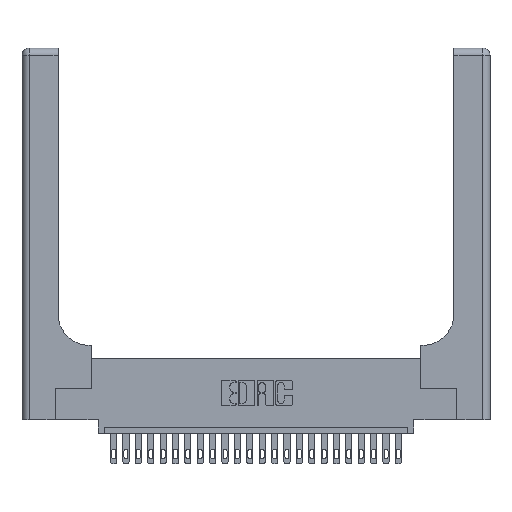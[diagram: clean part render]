
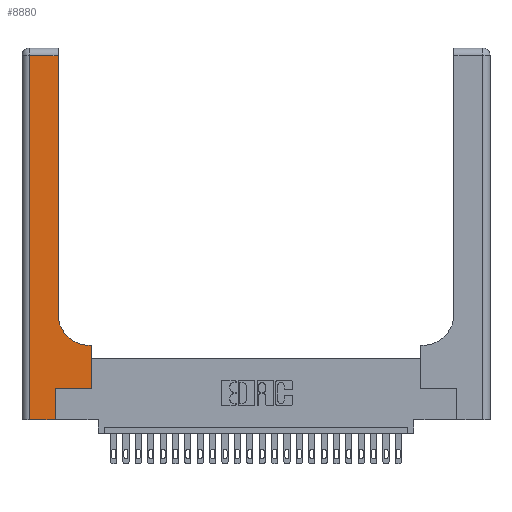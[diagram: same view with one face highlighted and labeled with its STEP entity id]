
A CAD part, top view. The second image highlights one B-rep face of the part: STEP entity #8880.
In plain terms, the highlighted planar face has unit normal (0, 0, 1).
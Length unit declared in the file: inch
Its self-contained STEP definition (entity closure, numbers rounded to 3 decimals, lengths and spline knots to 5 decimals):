
#120 = DIRECTION ( 'NONE',  ( 0., 1., 0. ) ) ;
#512 = ORIENTED_EDGE ( 'NONE', *, *, #14197, .T. ) ;
#911 = VERTEX_POINT ( 'NONE', #7799 ) ;
#1427 = LINE ( 'NONE', #4566, #17618 ) ;
#1475 = LINE ( 'NONE', #22172, #3324 ) ;
#1611 = PLANE ( 'NONE',  #11860 ) ;
#1965 = LINE ( 'NONE', #23813, #8492 ) ;
#2559 = LINE ( 'NONE', #25219, #19685 ) ;
#2937 = CARTESIAN_POINT ( 'NONE',  ( 0.269, 0., 0.37 ) ) ;
#3324 = VECTOR ( 'NONE', #23916, 39.37008 ) ;
#3340 = DIRECTION ( 'NONE',  ( 0., 1., 0. ) ) ;
#3597 = CARTESIAN_POINT ( 'NONE',  ( 0.06, 2.94, 0.37 ) ) ;
#3850 = VERTEX_POINT ( 'NONE', #7795 ) ;
#4311 = DIRECTION ( 'NONE',  ( -1., 0., 0. ) ) ;
#4566 = CARTESIAN_POINT ( 'NONE',  ( 0.5585, 0.25, 0.37 ) ) ;
#5113 = ORIENTED_EDGE ( 'NONE', *, *, #22026, .T. ) ;
#5158 = LINE ( 'NONE', #13811, #24402 ) ;
#5222 = VECTOR ( 'NONE', #4311, 39.37008 ) ;
#5595 = CARTESIAN_POINT ( 'NONE',  ( 0., 3., 0.37 ) ) ;
#5942 = VERTEX_POINT ( 'NONE', #2937 ) ;
#6068 = ORIENTED_EDGE ( 'NONE', *, *, #8853, .T. ) ;
#6918 = CARTESIAN_POINT ( 'NONE',  ( 0.2915, 2.94, 0.37 ) ) ;
#7169 = DIRECTION ( 'NONE',  ( 1., 0., 0. ) ) ;
#7316 = DIRECTION ( 'NONE',  ( 1., 0., 0. ) ) ;
#7342 = VERTEX_POINT ( 'NONE', #24011 ) ;
#7644 = ORIENTED_EDGE ( 'NONE', *, *, #8374, .T. ) ;
#7795 = CARTESIAN_POINT ( 'NONE',  ( 0.5585, 0.25, 0.37 ) ) ;
#7799 = CARTESIAN_POINT ( 'NONE',  ( 0.06, 0., 0.37 ) ) ;
#8374 = EDGE_CURVE ( 'NONE', #11937, #13848, #12466, .T. ) ;
#8492 = VECTOR ( 'NONE', #14011, 39.37008 ) ;
#8853 = EDGE_CURVE ( 'NONE', #5942, #13074, #2559, .T. ) ;
#8880 = ADVANCED_FACE ( 'NONE', ( #17200 ), #1611, .F. ) ;
#8894 = ORIENTED_EDGE ( 'NONE', *, *, #12734, .T. ) ;
#9008 = EDGE_CURVE ( 'NONE', #13074, #3850, #12842, .T. ) ;
#9330 = VECTOR ( 'NONE', #24207, 39.37008 ) ;
#9724 = ORIENTED_EDGE ( 'NONE', *, *, #12870, .T. ) ;
#11233 = EDGE_LOOP ( 'NONE', ( #8894, #5113, #18262, #512, #6068, #13697, #9724, #7644, #15620 ) ) ;
#11236 = CARTESIAN_POINT ( 'NONE',  ( 0.5585, 0.6, 0.37 ) ) ;
#11566 = DIRECTION ( 'NONE',  ( 0., 0., -1. ) ) ;
#11860 = AXIS2_PLACEMENT_3D ( 'NONE', #5595, #13431, #17603 ) ;
#11937 = VERTEX_POINT ( 'NONE', #11236 ) ;
#12322 = CARTESIAN_POINT ( 'NONE',  ( 0.2915, 0.6, 0.37 ) ) ;
#12466 = LINE ( 'NONE', #12322, #9330 ) ;
#12555 = CIRCLE ( 'NONE', #24751, 0.25 ) ;
#12734 = EDGE_CURVE ( 'NONE', #7342, #16604, #5158, .T. ) ;
#12842 = LINE ( 'NONE', #16799, #15008 ) ;
#12870 = EDGE_CURVE ( 'NONE', #3850, #11937, #1427, .T. ) ;
#13074 = VERTEX_POINT ( 'NONE', #19001 ) ;
#13431 = DIRECTION ( 'NONE',  ( 0., 0., -1. ) ) ;
#13697 = ORIENTED_EDGE ( 'NONE', *, *, #9008, .T. ) ;
#13811 = CARTESIAN_POINT ( 'NONE',  ( 0.2915, 3., 0.37 ) ) ;
#13848 = VERTEX_POINT ( 'NONE', #18695 ) ;
#13914 = LINE ( 'NONE', #21549, #5222 ) ;
#14011 = DIRECTION ( 'NONE',  ( 1., 0., 0. ) ) ;
#14156 = VERTEX_POINT ( 'NONE', #3597 ) ;
#14197 = EDGE_CURVE ( 'NONE', #911, #5942, #1965, .T. ) ;
#15008 = VECTOR ( 'NONE', #7169, 39.37008 ) ;
#15620 = ORIENTED_EDGE ( 'NONE', *, *, #25068, .T. ) ;
#16273 = EDGE_CURVE ( 'NONE', #14156, #911, #1475, .T. ) ;
#16292 = DIRECTION ( 'NONE',  ( 0., 1., 0. ) ) ;
#16604 = VERTEX_POINT ( 'NONE', #6918 ) ;
#16799 = CARTESIAN_POINT ( 'NONE',  ( 0.269, 0.25, 0.37 ) ) ;
#17200 = FACE_OUTER_BOUND ( 'NONE', #11233, .T. ) ;
#17603 = DIRECTION ( 'NONE',  ( -1., 0., 0. ) ) ;
#17618 = VECTOR ( 'NONE', #16292, 39.37008 ) ;
#18262 = ORIENTED_EDGE ( 'NONE', *, *, #16273, .T. ) ;
#18695 = CARTESIAN_POINT ( 'NONE',  ( 0.5415, 0.6, 0.37 ) ) ;
#19001 = CARTESIAN_POINT ( 'NONE',  ( 0.269, 0.25, 0.37 ) ) ;
#19685 = VECTOR ( 'NONE', #3340, 39.37008 ) ;
#21118 = CARTESIAN_POINT ( 'NONE',  ( 0.5415, 0.85, 0.37 ) ) ;
#21549 = CARTESIAN_POINT ( 'NONE',  ( 0., 2.94, 0.37 ) ) ;
#22026 = EDGE_CURVE ( 'NONE', #16604, #14156, #13914, .T. ) ;
#22172 = CARTESIAN_POINT ( 'NONE',  ( 0.06, 3., 0.37 ) ) ;
#23813 = CARTESIAN_POINT ( 'NONE',  ( 0., 0., 0.37 ) ) ;
#23916 = DIRECTION ( 'NONE',  ( 0., -1., 0. ) ) ;
#24011 = CARTESIAN_POINT ( 'NONE',  ( 0.2915, 0.85, 0.37 ) ) ;
#24207 = DIRECTION ( 'NONE',  ( -1., 0., 0. ) ) ;
#24402 = VECTOR ( 'NONE', #120, 39.37008 ) ;
#24751 = AXIS2_PLACEMENT_3D ( 'NONE', #21118, #11566, #7316 ) ;
#25068 = EDGE_CURVE ( 'NONE', #13848, #7342, #12555, .T. ) ;
#25219 = CARTESIAN_POINT ( 'NONE',  ( 0.269, 0., 0.37 ) ) ;
